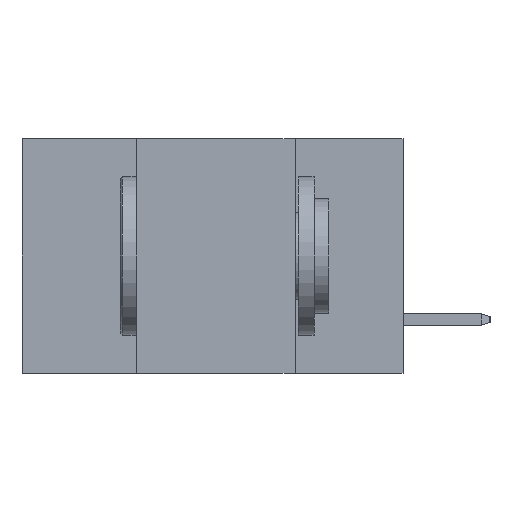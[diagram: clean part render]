
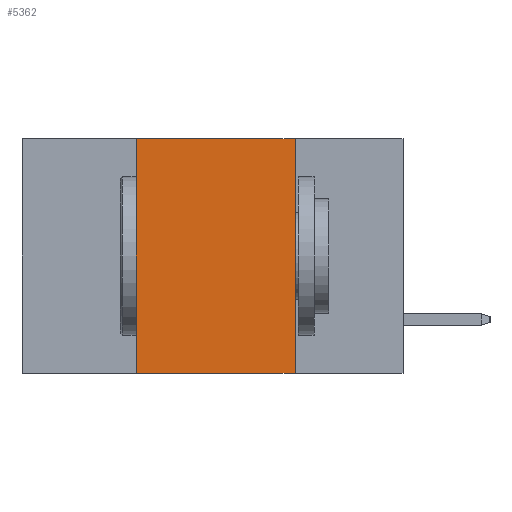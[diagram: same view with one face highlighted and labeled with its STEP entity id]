
A CAD part, left-side view. The second image highlights one B-rep face of the part: STEP entity #5362.
In plain terms, the highlighted planar face has unit normal (-1, 0, 0).
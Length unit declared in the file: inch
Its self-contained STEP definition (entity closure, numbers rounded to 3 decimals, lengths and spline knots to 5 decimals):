
#277 = LINE ( 'NONE', #7129, #3475 ) ;
#1022 = VECTOR ( 'NONE', #8987, 39.37008 ) ;
#1319 = FACE_OUTER_BOUND ( 'NONE', #7750, .T. ) ;
#1931 = CARTESIAN_POINT ( 'NONE',  ( 0., 0.17, -0.37 ) ) ;
#2174 = ORIENTED_EDGE ( 'NONE', *, *, #10241, .T. ) ;
#2180 = DIRECTION ( 'NONE',  ( 0., -1., 0. ) ) ;
#2239 = LINE ( 'NONE', #9590, #4056 ) ;
#3027 = PLANE ( 'NONE',  #9857 ) ;
#3138 = DIRECTION ( 'NONE',  ( 1., 0., 0. ) ) ;
#3457 = VERTEX_POINT ( 'NONE', #7959 ) ;
#3475 = VECTOR ( 'NONE', #6079, 39.37008 ) ;
#4056 = VECTOR ( 'NONE', #2180, 39.37008 ) ;
#4489 = EDGE_CURVE ( 'NONE', #6773, #3457, #2239, .T. ) ;
#4681 = CARTESIAN_POINT ( 'NONE',  ( 0., 0.17, 0. ) ) ;
#4698 = LINE ( 'NONE', #8064, #1022 ) ;
#5362 = ADVANCED_FACE ( 'NONE', ( #1319 ), #3027, .F. ) ;
#5411 = CARTESIAN_POINT ( 'NONE',  ( 0., 0.42, -0.37 ) ) ;
#5420 = ORIENTED_EDGE ( 'NONE', *, *, #8740, .F. ) ;
#6079 = DIRECTION ( 'NONE',  ( 0., 0., 1. ) ) ;
#6363 = DIRECTION ( 'NONE',  ( 0., 0., -1. ) ) ;
#6520 = ORIENTED_EDGE ( 'NONE', *, *, #6672, .F. ) ;
#6672 = EDGE_CURVE ( 'NONE', #3457, #9901, #8868, .T. ) ;
#6773 = VERTEX_POINT ( 'NONE', #9124 ) ;
#7129 = CARTESIAN_POINT ( 'NONE',  ( 0., 0.42, 0. ) ) ;
#7450 = ORIENTED_EDGE ( 'NONE', *, *, #4489, .F. ) ;
#7750 = EDGE_LOOP ( 'NONE', ( #6520, #7450, #5420, #2174 ) ) ;
#7959 = CARTESIAN_POINT ( 'NONE',  ( 0., 0.17, 0. ) ) ;
#8064 = CARTESIAN_POINT ( 'NONE',  ( 0., 0.6, -0.37 ) ) ;
#8143 = VECTOR ( 'NONE', #8967, 39.37008 ) ;
#8740 = EDGE_CURVE ( 'NONE', #9125, #6773, #277, .T. ) ;
#8868 = LINE ( 'NONE', #4681, #8143 ) ;
#8951 = CARTESIAN_POINT ( 'NONE',  ( 0., 0.6, 0. ) ) ;
#8967 = DIRECTION ( 'NONE',  ( 0., 0., -1. ) ) ;
#8987 = DIRECTION ( 'NONE',  ( 0., -1., 0. ) ) ;
#9124 = CARTESIAN_POINT ( 'NONE',  ( 0., 0.42, 0. ) ) ;
#9125 = VERTEX_POINT ( 'NONE', #5411 ) ;
#9590 = CARTESIAN_POINT ( 'NONE',  ( 0., 0.6, 0. ) ) ;
#9857 = AXIS2_PLACEMENT_3D ( 'NONE', #8951, #3138, #6363 ) ;
#9901 = VERTEX_POINT ( 'NONE', #1931 ) ;
#10241 = EDGE_CURVE ( 'NONE', #9125, #9901, #4698, .T. ) ;
